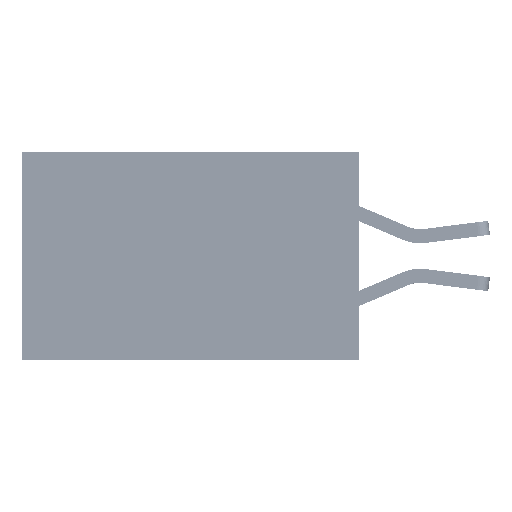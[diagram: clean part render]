
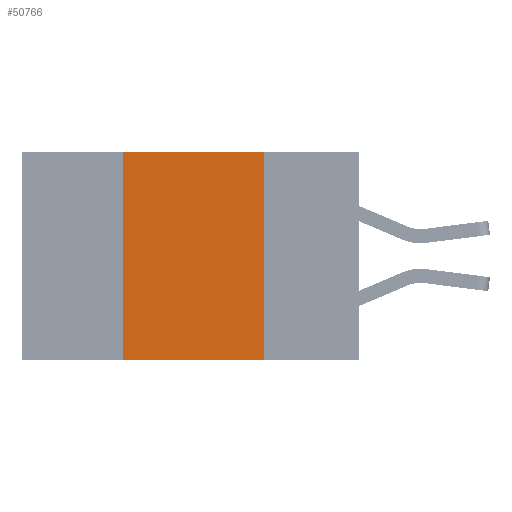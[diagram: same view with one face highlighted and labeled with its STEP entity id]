
A CAD part, left-side view. The second image highlights one B-rep face of the part: STEP entity #50766.
In plain terms, the highlighted planar face has unit normal (-1, 0, 0).
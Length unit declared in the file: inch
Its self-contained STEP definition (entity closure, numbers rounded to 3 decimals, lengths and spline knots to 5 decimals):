
#1384 = VECTOR ( 'NONE', #38273, 39.37008 ) ;
#4127 = VECTOR ( 'NONE', #33376, 39.37008 ) ;
#4648 = CARTESIAN_POINT ( 'NONE',  ( 0., 0.42, -0.37 ) ) ;
#5066 = VECTOR ( 'NONE', #12989, 39.37008 ) ;
#5359 = DIRECTION ( 'NONE',  ( 0., 0., -1. ) ) ;
#5452 = DIRECTION ( 'NONE',  ( 0., -1., 0. ) ) ;
#9090 = CARTESIAN_POINT ( 'NONE',  ( 0., 0.42, 0. ) ) ;
#9344 = DIRECTION ( 'NONE',  ( 1., 0., 0. ) ) ;
#9430 = ORIENTED_EDGE ( 'NONE', *, *, #52589, .F. ) ;
#10933 = EDGE_CURVE ( 'NONE', #11327, #32080, #24997, .T. ) ;
#11327 = VERTEX_POINT ( 'NONE', #47649 ) ;
#12989 = DIRECTION ( 'NONE',  ( 0., 0., -1. ) ) ;
#14243 = CARTESIAN_POINT ( 'NONE',  ( 0., 0.6, -0.37 ) ) ;
#16850 = LINE ( 'NONE', #49410, #4127 ) ;
#20994 = CARTESIAN_POINT ( 'NONE',  ( 0., 0.17, 0. ) ) ;
#21990 = LINE ( 'NONE', #14243, #38374 ) ;
#22145 = PLANE ( 'NONE',  #49853 ) ;
#24627 = ORIENTED_EDGE ( 'NONE', *, *, #38885, .F. ) ;
#24997 = LINE ( 'NONE', #20994, #5066 ) ;
#26672 = VERTEX_POINT ( 'NONE', #9090 ) ;
#26777 = LINE ( 'NONE', #43058, #1384 ) ;
#30610 = VERTEX_POINT ( 'NONE', #4648 ) ;
#30917 = ORIENTED_EDGE ( 'NONE', *, *, #10933, .F. ) ;
#32080 = VERTEX_POINT ( 'NONE', #35530 ) ;
#33376 = DIRECTION ( 'NONE',  ( 0., -1., 0. ) ) ;
#33637 = CARTESIAN_POINT ( 'NONE',  ( 0., 0.6, 0. ) ) ;
#35305 = ORIENTED_EDGE ( 'NONE', *, *, #43892, .T. ) ;
#35530 = CARTESIAN_POINT ( 'NONE',  ( 0., 0.17, -0.37 ) ) ;
#38273 = DIRECTION ( 'NONE',  ( 0., 0., 1. ) ) ;
#38374 = VECTOR ( 'NONE', #5452, 39.37008 ) ;
#38885 = EDGE_CURVE ( 'NONE', #26672, #11327, #16850, .T. ) ;
#41914 = FACE_OUTER_BOUND ( 'NONE', #51185, .T. ) ;
#43058 = CARTESIAN_POINT ( 'NONE',  ( 0., 0.42, 0. ) ) ;
#43892 = EDGE_CURVE ( 'NONE', #30610, #32080, #21990, .T. ) ;
#47649 = CARTESIAN_POINT ( 'NONE',  ( 0., 0.17, 0. ) ) ;
#49410 = CARTESIAN_POINT ( 'NONE',  ( 0., 0.6, 0. ) ) ;
#49853 = AXIS2_PLACEMENT_3D ( 'NONE', #33637, #9344, #5359 ) ;
#50766 = ADVANCED_FACE ( 'NONE', ( #41914 ), #22145, .F. ) ;
#51185 = EDGE_LOOP ( 'NONE', ( #30917, #24627, #9430, #35305 ) ) ;
#52589 = EDGE_CURVE ( 'NONE', #30610, #26672, #26777, .T. ) ;
